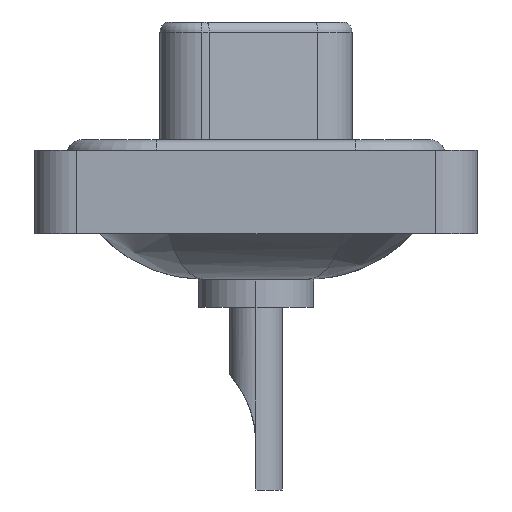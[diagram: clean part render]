
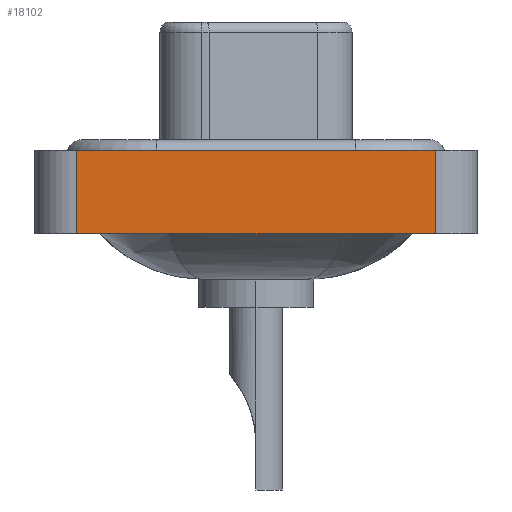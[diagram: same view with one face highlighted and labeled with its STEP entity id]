
A CAD part, left-side view. The second image highlights one B-rep face of the part: STEP entity #18102.
In plain terms, the highlighted planar face has unit normal (-1, 0, 0).
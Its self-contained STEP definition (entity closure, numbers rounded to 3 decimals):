
#97 = LINE ( 'NONE', #9119, #11165 ) ;
#677 = CARTESIAN_POINT ( 'NONE',  ( -7.3, 8.55, 0.4 ) ) ;
#902 = CARTESIAN_POINT ( 'NONE',  ( -7.3, 8.55, -3.6 ) ) ;
#1111 = DIRECTION ( 'NONE',  ( -1., 0., 0. ) ) ;
#1332 = LINE ( 'NONE', #10139, #19116 ) ;
#1495 = DIRECTION ( 'NONE',  ( 0., -1., 0. ) ) ;
#2059 = EDGE_CURVE ( 'NONE', #6999, #17142, #14434, .T. ) ;
#2972 = CARTESIAN_POINT ( 'NONE',  ( -7.3, -8.55, 0.4 ) ) ;
#3279 = EDGE_LOOP ( 'NONE', ( #7749, #8768, #8640, #11757 ) ) ;
#6999 = VERTEX_POINT ( 'NONE', #12564 ) ;
#7749 = ORIENTED_EDGE ( 'NONE', *, *, #11965, .T. ) ;
#8569 = CARTESIAN_POINT ( 'NONE',  ( -7.3, -8.55, -3.6 ) ) ;
#8640 = ORIENTED_EDGE ( 'NONE', *, *, #2059, .F. ) ;
#8723 = EDGE_CURVE ( 'NONE', #17142, #15674, #10472, .T. ) ;
#8768 = ORIENTED_EDGE ( 'NONE', *, *, #8723, .F. ) ;
#9119 = CARTESIAN_POINT ( 'NONE',  ( -7.3, -8.55, -3.6 ) ) ;
#9589 = EDGE_CURVE ( 'NONE', #6999, #16357, #97, .T. ) ;
#10139 = CARTESIAN_POINT ( 'NONE',  ( -7.3, -8.55, -3.6 ) ) ;
#10472 = LINE ( 'NONE', #2972, #16173 ) ;
#11165 = VECTOR ( 'NONE', #1495, 1000. ) ;
#11481 = DIRECTION ( 'NONE',  ( 0., 0., 1. ) ) ;
#11757 = ORIENTED_EDGE ( 'NONE', *, *, #9589, .T. ) ;
#11965 = EDGE_CURVE ( 'NONE', #16357, #15674, #1332, .T. ) ;
#12236 = VECTOR ( 'NONE', #11481, 1000. ) ;
#12564 = CARTESIAN_POINT ( 'NONE',  ( -7.3, 8.55, -3.6 ) ) ;
#13581 = AXIS2_PLACEMENT_3D ( 'NONE', #19000, #1111, #17509 ) ;
#14349 = PLANE ( 'NONE',  #13581 ) ;
#14434 = LINE ( 'NONE', #902, #12236 ) ;
#15101 = DIRECTION ( 'NONE',  ( 0., -1., 0. ) ) ;
#15674 = VERTEX_POINT ( 'NONE', #16975 ) ;
#16173 = VECTOR ( 'NONE', #15101, 1000. ) ;
#16357 = VERTEX_POINT ( 'NONE', #8569 ) ;
#16975 = CARTESIAN_POINT ( 'NONE',  ( -7.3, -8.55, 0.4 ) ) ;
#17142 = VERTEX_POINT ( 'NONE', #677 ) ;
#17408 = FACE_OUTER_BOUND ( 'NONE', #3279, .T. ) ;
#17509 = DIRECTION ( 'NONE',  ( 0., 0., 1. ) ) ;
#17828 = DIRECTION ( 'NONE',  ( 0., 0., 1. ) ) ;
#18102 = ADVANCED_FACE ( 'NONE', ( #17408 ), #14349, .T. ) ;
#19000 = CARTESIAN_POINT ( 'NONE',  ( -7.3, -8.55, -3.6 ) ) ;
#19116 = VECTOR ( 'NONE', #17828, 1000. ) ;
